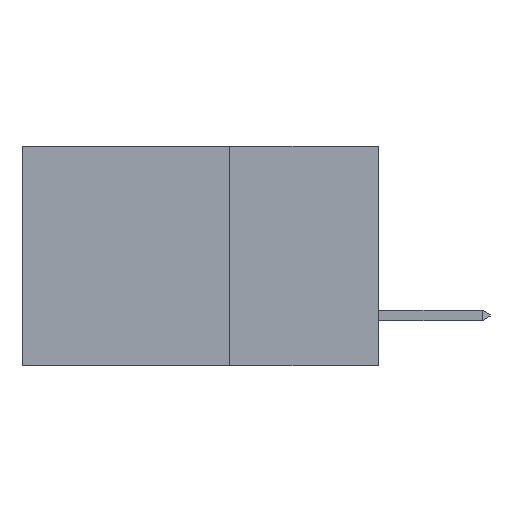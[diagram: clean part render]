
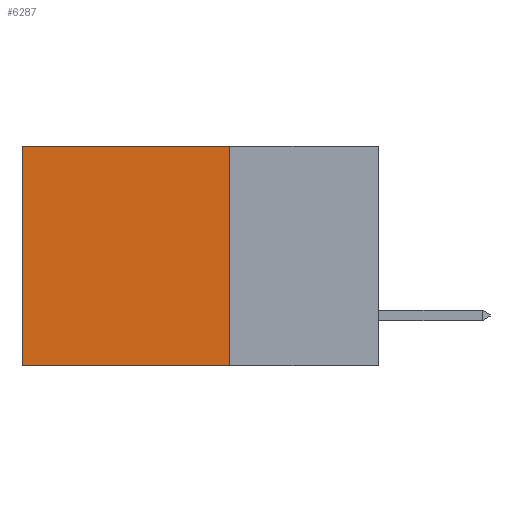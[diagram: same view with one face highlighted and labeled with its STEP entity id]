
A CAD part, left-side view. The second image highlights one B-rep face of the part: STEP entity #6287.
In plain terms, the highlighted planar face has unit normal (-1, 0, 0).
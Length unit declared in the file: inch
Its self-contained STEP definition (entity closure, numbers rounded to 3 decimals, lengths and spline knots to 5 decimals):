
#1202 = EDGE_LOOP ( 'NONE', ( #5978, #4035, #6278, #4273 ) ) ;
#1436 = LINE ( 'NONE', #10840, #5496 ) ;
#1472 = CARTESIAN_POINT ( 'NONE',  ( 0.2615, 0.25, 0. ) ) ;
#1673 = VERTEX_POINT ( 'NONE', #9213 ) ;
#1994 = VERTEX_POINT ( 'NONE', #9604 ) ;
#2378 = AXIS2_PLACEMENT_3D ( 'NONE', #8782, #8481, #8470 ) ;
#2674 = CARTESIAN_POINT ( 'NONE',  ( 0.2615, 0.6, -0.37 ) ) ;
#3496 = DIRECTION ( 'NONE',  ( 0., 0., -1. ) ) ;
#3579 = FACE_OUTER_BOUND ( 'NONE', #1202, .T. ) ;
#3996 = VECTOR ( 'NONE', #6692, 39.37008 ) ;
#4035 = ORIENTED_EDGE ( 'NONE', *, *, #4888, .F. ) ;
#4273 = ORIENTED_EDGE ( 'NONE', *, *, #9815, .T. ) ;
#4512 = VECTOR ( 'NONE', #3496, 39.37008 ) ;
#4753 = LINE ( 'NONE', #2674, #4512 ) ;
#4888 = EDGE_CURVE ( 'NONE', #5708, #1673, #7793, .T. ) ;
#5354 = VECTOR ( 'NONE', #8627, 39.37008 ) ;
#5496 = VECTOR ( 'NONE', #10035, 39.37008 ) ;
#5708 = VERTEX_POINT ( 'NONE', #5952 ) ;
#5746 = CARTESIAN_POINT ( 'NONE',  ( 0.2615, 0.25, -0.37 ) ) ;
#5952 = CARTESIAN_POINT ( 'NONE',  ( 0.2615, 0.25, -0.37 ) ) ;
#5978 = ORIENTED_EDGE ( 'NONE', *, *, #8436, .T. ) ;
#6227 = LINE ( 'NONE', #5746, #3996 ) ;
#6278 = ORIENTED_EDGE ( 'NONE', *, *, #10555, .F. ) ;
#6287 = ADVANCED_FACE ( 'NONE', ( #3579 ), #8546, .F. ) ;
#6608 = VERTEX_POINT ( 'NONE', #1472 ) ;
#6692 = DIRECTION ( 'NONE',  ( 0., 0., -1. ) ) ;
#7793 = LINE ( 'NONE', #10630, #5354 ) ;
#8436 = EDGE_CURVE ( 'NONE', #1994, #1673, #4753, .T. ) ;
#8470 = DIRECTION ( 'NONE',  ( 0., 0., -1. ) ) ;
#8481 = DIRECTION ( 'NONE',  ( 1., 0., 0. ) ) ;
#8546 = PLANE ( 'NONE',  #2378 ) ;
#8627 = DIRECTION ( 'NONE',  ( 0., 1., 0. ) ) ;
#8782 = CARTESIAN_POINT ( 'NONE',  ( 0.2615, 0.25, -0.37 ) ) ;
#9213 = CARTESIAN_POINT ( 'NONE',  ( 0.2615, 0.6, -0.37 ) ) ;
#9604 = CARTESIAN_POINT ( 'NONE',  ( 0.2615, 0.6, 0. ) ) ;
#9815 = EDGE_CURVE ( 'NONE', #6608, #1994, #1436, .T. ) ;
#10035 = DIRECTION ( 'NONE',  ( 0., 1., 0. ) ) ;
#10555 = EDGE_CURVE ( 'NONE', #6608, #5708, #6227, .T. ) ;
#10630 = CARTESIAN_POINT ( 'NONE',  ( 0.2615, 0.25, -0.37 ) ) ;
#10840 = CARTESIAN_POINT ( 'NONE',  ( 0.2615, 0.25, 0. ) ) ;
